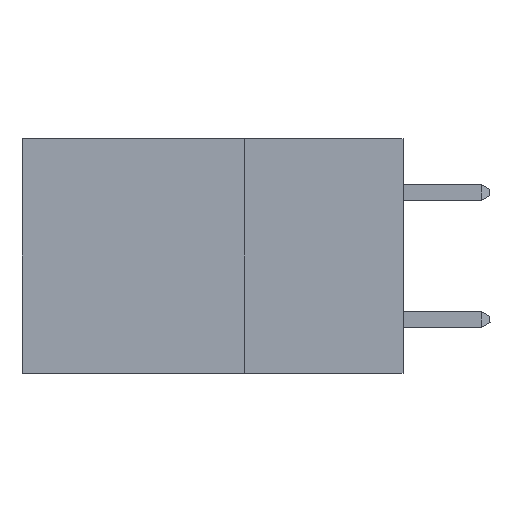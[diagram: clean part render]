
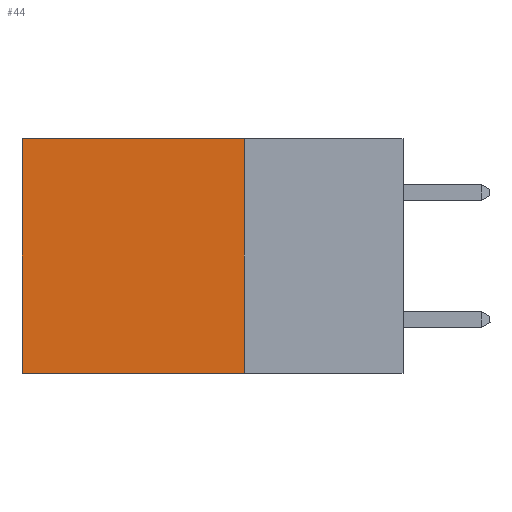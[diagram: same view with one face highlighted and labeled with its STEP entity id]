
A CAD part, left-side view. The second image highlights one B-rep face of the part: STEP entity #44.
In plain terms, the highlighted planar face has unit normal (-1, 0, 0).
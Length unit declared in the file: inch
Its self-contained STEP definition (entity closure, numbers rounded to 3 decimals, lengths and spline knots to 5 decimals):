
#6 = EDGE_CURVE ( 'NONE', #5683, #2748, #3527, .T. ) ;
#44 = ADVANCED_FACE ( 'NONE', ( #1335 ), #185, .F. ) ;
#156 = EDGE_CURVE ( 'NONE', #3169, #2748, #7721, .T. ) ;
#185 = PLANE ( 'NONE',  #8046 ) ;
#240 = EDGE_CURVE ( 'NONE', #1198, #5683, #3540, .T. ) ;
#440 = VECTOR ( 'NONE', #4354, 39.37008 ) ;
#1198 = VERTEX_POINT ( 'NONE', #6552 ) ;
#1209 = EDGE_LOOP ( 'NONE', ( #7450, #6976, #8833, #6155 ) ) ;
#1335 = FACE_OUTER_BOUND ( 'NONE', #1209, .T. ) ;
#2412 = CARTESIAN_POINT ( 'NONE',  ( 0.2875, 0.6, 0. ) ) ;
#2748 = VERTEX_POINT ( 'NONE', #8250 ) ;
#2786 = VECTOR ( 'NONE', #5910, 39.37008 ) ;
#3169 = VERTEX_POINT ( 'NONE', #6074 ) ;
#3518 = EDGE_CURVE ( 'NONE', #1198, #3169, #7819, .T. ) ;
#3527 = LINE ( 'NONE', #4593, #5360 ) ;
#3540 = LINE ( 'NONE', #8099, #8629 ) ;
#4217 = DIRECTION ( 'NONE',  ( 0., 1., 0. ) ) ;
#4354 = DIRECTION ( 'NONE',  ( 0., 0., -1. ) ) ;
#4487 = CARTESIAN_POINT ( 'NONE',  ( 0.2875, 0.25, 0. ) ) ;
#4593 = CARTESIAN_POINT ( 'NONE',  ( 0.2875, 0.6, 0. ) ) ;
#4837 = DIRECTION ( 'NONE',  ( 0., 0., -1. ) ) ;
#5143 = DIRECTION ( 'NONE',  ( 0., 0., -1. ) ) ;
#5147 = DIRECTION ( 'NONE',  ( 1., 0., 0. ) ) ;
#5215 = CARTESIAN_POINT ( 'NONE',  ( 0.2875, 0.25, 0. ) ) ;
#5360 = VECTOR ( 'NONE', #4837, 39.37008 ) ;
#5683 = VERTEX_POINT ( 'NONE', #2412 ) ;
#5910 = DIRECTION ( 'NONE',  ( 0., 1., 0. ) ) ;
#6074 = CARTESIAN_POINT ( 'NONE',  ( 0.2875, 0.25, -0.37 ) ) ;
#6155 = ORIENTED_EDGE ( 'NONE', *, *, #240, .T. ) ;
#6552 = CARTESIAN_POINT ( 'NONE',  ( 0.2875, 0.25, 0. ) ) ;
#6976 = ORIENTED_EDGE ( 'NONE', *, *, #156, .F. ) ;
#7450 = ORIENTED_EDGE ( 'NONE', *, *, #6, .T. ) ;
#7721 = LINE ( 'NONE', #8398, #2786 ) ;
#7819 = LINE ( 'NONE', #4487, #440 ) ;
#8046 = AXIS2_PLACEMENT_3D ( 'NONE', #5215, #5147, #5143 ) ;
#8099 = CARTESIAN_POINT ( 'NONE',  ( 0.2875, 0.25, 0. ) ) ;
#8250 = CARTESIAN_POINT ( 'NONE',  ( 0.2875, 0.6, -0.37 ) ) ;
#8398 = CARTESIAN_POINT ( 'NONE',  ( 0.2875, 0.25, -0.37 ) ) ;
#8629 = VECTOR ( 'NONE', #4217, 39.37008 ) ;
#8833 = ORIENTED_EDGE ( 'NONE', *, *, #3518, .F. ) ;
